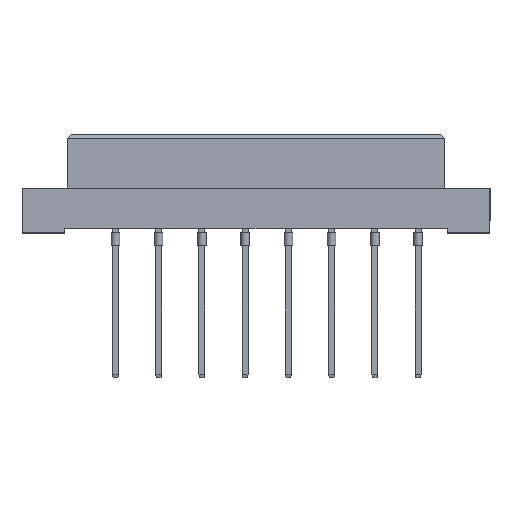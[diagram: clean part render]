
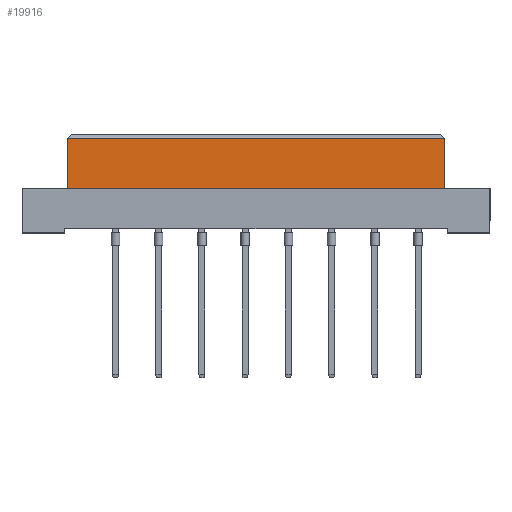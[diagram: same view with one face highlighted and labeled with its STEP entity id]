
A CAD part, top view. The second image highlights one B-rep face of the part: STEP entity #19916.
In plain terms, the highlighted planar face has unit normal (0, 0, 1).
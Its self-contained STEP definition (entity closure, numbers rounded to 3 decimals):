
#631 = DIRECTION ( 'NONE',  ( 1., 0., 0. ) ) ;
#764 = EDGE_CURVE ( 'NONE', #9895, #3875, #15646, .T. ) ;
#1255 = LINE ( 'NONE', #7883, #14375 ) ;
#2209 = LINE ( 'NONE', #5350, #8841 ) ;
#2851 = DIRECTION ( 'NONE',  ( 1., 0., 0. ) ) ;
#3592 = CARTESIAN_POINT ( 'NONE',  ( 22.2, -0.5, 4.25 ) ) ;
#3875 = VERTEX_POINT ( 'NONE', #4866 ) ;
#4866 = CARTESIAN_POINT ( 'NONE',  ( -22.2, -0.5, 4.25 ) ) ;
#5350 = CARTESIAN_POINT ( 'NONE',  ( 22.2, -6.4, 4.25 ) ) ;
#6860 = VECTOR ( 'NONE', #13215, 1000. ) ;
#7883 = CARTESIAN_POINT ( 'NONE',  ( 22.2, -6.4, 4.25 ) ) ;
#8086 = ORIENTED_EDGE ( 'NONE', *, *, #10400, .T. ) ;
#8678 = VERTEX_POINT ( 'NONE', #20576 ) ;
#8841 = VECTOR ( 'NONE', #631, 1000. ) ;
#9790 = AXIS2_PLACEMENT_3D ( 'NONE', #18722, #10838, #2851 ) ;
#9895 = VERTEX_POINT ( 'NONE', #3592 ) ;
#10324 = ORIENTED_EDGE ( 'NONE', *, *, #764, .T. ) ;
#10376 = EDGE_CURVE ( 'NONE', #16785, #3875, #18174, .T. ) ;
#10400 = EDGE_CURVE ( 'NONE', #16785, #8678, #2209, .T. ) ;
#10838 = DIRECTION ( 'NONE',  ( 0., 0., 1. ) ) ;
#10929 = CARTESIAN_POINT ( 'NONE',  ( -22.2, -0.5, 4.25 ) ) ;
#11327 = EDGE_LOOP ( 'NONE', ( #13131, #10324, #13366, #8086 ) ) ;
#12560 = VECTOR ( 'NONE', #16608, 1000. ) ;
#13131 = ORIENTED_EDGE ( 'NONE', *, *, #13497, .T. ) ;
#13215 = DIRECTION ( 'NONE',  ( -1., 0., 0. ) ) ;
#13366 = ORIENTED_EDGE ( 'NONE', *, *, #10376, .F. ) ;
#13497 = EDGE_CURVE ( 'NONE', #8678, #9895, #1255, .T. ) ;
#14304 = DIRECTION ( 'NONE',  ( 0., 1., 0. ) ) ;
#14375 = VECTOR ( 'NONE', #14304, 1000. ) ;
#15014 = CARTESIAN_POINT ( 'NONE',  ( -22.2, -6.4, 4.25 ) ) ;
#15460 = PLANE ( 'NONE',  #9790 ) ;
#15646 = LINE ( 'NONE', #10929, #6860 ) ;
#16608 = DIRECTION ( 'NONE',  ( 0., 1., 0. ) ) ;
#16785 = VERTEX_POINT ( 'NONE', #15014 ) ;
#18174 = LINE ( 'NONE', #18290, #12560 ) ;
#18290 = CARTESIAN_POINT ( 'NONE',  ( -22.2, -6.4, 4.25 ) ) ;
#18722 = CARTESIAN_POINT ( 'NONE',  ( 22.2, -6.4, 4.25 ) ) ;
#18820 = FACE_OUTER_BOUND ( 'NONE', #11327, .T. ) ;
#19916 = ADVANCED_FACE ( 'NONE', ( #18820 ), #15460, .T. ) ;
#20576 = CARTESIAN_POINT ( 'NONE',  ( 22.2, -6.4, 4.25 ) ) ;
